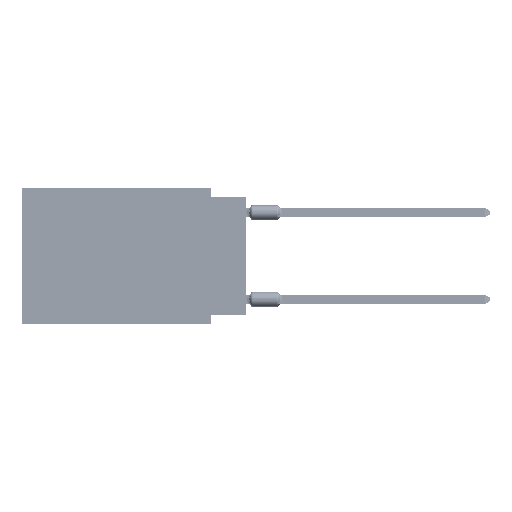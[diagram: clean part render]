
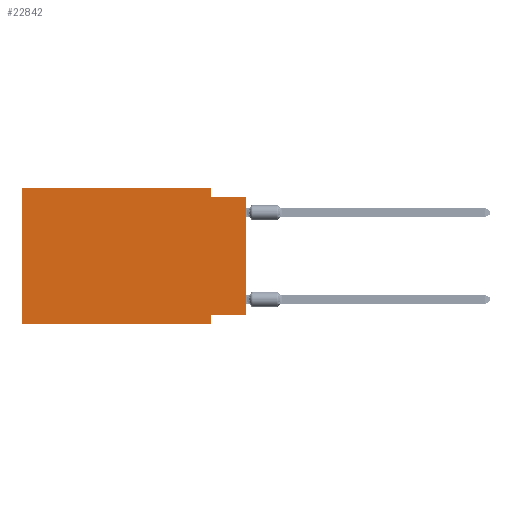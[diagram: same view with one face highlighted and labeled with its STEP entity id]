
A CAD part, left-side view. The second image highlights one B-rep face of the part: STEP entity #22842.
In plain terms, the highlighted planar face has unit normal (-1, 0, 0).
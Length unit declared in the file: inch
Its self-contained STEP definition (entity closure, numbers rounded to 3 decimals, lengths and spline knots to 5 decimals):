
#12 = VERTEX_POINT ( 'NONE', #15756 ) ;
#112 = FACE_OUTER_BOUND ( 'NONE', #55734, .T. ) ;
#327 = EDGE_CURVE ( 'NONE', #12, #71930, #74552, .T. ) ;
#1677 = DIRECTION ( 'NONE',  ( 0., 0., -1. ) ) ;
#2386 = ORIENTED_EDGE ( 'NONE', *, *, #60859, .T. ) ;
#9973 = CARTESIAN_POINT ( 'NONE',  ( 0., 0.645, -0.39 ) ) ;
#10637 = CARTESIAN_POINT ( 'NONE',  ( 0., 0.1, 0. ) ) ;
#10812 = VECTOR ( 'NONE', #62436, 39.37008 ) ;
#10823 = EDGE_CURVE ( 'NONE', #30338, #66851, #62764, .T. ) ;
#11741 = LINE ( 'NONE', #49872, #10812 ) ;
#14947 = CARTESIAN_POINT ( 'NONE',  ( 0., 0.645, 0. ) ) ;
#15350 = LINE ( 'NONE', #14947, #48545 ) ;
#15441 = VECTOR ( 'NONE', #75757, 39.37008 ) ;
#15746 = ORIENTED_EDGE ( 'NONE', *, *, #327, .F. ) ;
#15756 = CARTESIAN_POINT ( 'NONE',  ( 0., 0.1, -0.025 ) ) ;
#17090 = EDGE_CURVE ( 'NONE', #29389, #30338, #11741, .T. ) ;
#18115 = LINE ( 'NONE', #48184, #34648 ) ;
#18523 = EDGE_CURVE ( 'NONE', #76039, #56901, #15350, .T. ) ;
#19730 = CARTESIAN_POINT ( 'NONE',  ( 0., 0.1, -0.365 ) ) ;
#22842 = ADVANCED_FACE ( 'NONE', ( #112 ), #74008, .F. ) ;
#25514 = CARTESIAN_POINT ( 'NONE',  ( 0., 0.645, 0. ) ) ;
#29389 = VERTEX_POINT ( 'NONE', #50410 ) ;
#30338 = VERTEX_POINT ( 'NONE', #19730 ) ;
#30595 = CARTESIAN_POINT ( 'NONE',  ( 0., 0.645, -0.39 ) ) ;
#31672 = CARTESIAN_POINT ( 'NONE',  ( 0., 0.645, 0. ) ) ;
#32279 = EDGE_CURVE ( 'NONE', #56901, #12, #40653, .T. ) ;
#32532 = CARTESIAN_POINT ( 'NONE',  ( 0., 0.1, 0. ) ) ;
#33145 = VECTOR ( 'NONE', #62234, 39.37008 ) ;
#34553 = AXIS2_PLACEMENT_3D ( 'NONE', #41994, #73611, #61027 ) ;
#34648 = VECTOR ( 'NONE', #55455, 39.37008 ) ;
#34811 = CARTESIAN_POINT ( 'NONE',  ( 0., 0.1, -0.39 ) ) ;
#35458 = VECTOR ( 'NONE', #62369, 39.37008 ) ;
#40653 = LINE ( 'NONE', #32532, #79321 ) ;
#41693 = VERTEX_POINT ( 'NONE', #9973 ) ;
#41994 = CARTESIAN_POINT ( 'NONE',  ( 0., 0.645, 0. ) ) ;
#43728 = CARTESIAN_POINT ( 'NONE',  ( 0., 0., -0.025 ) ) ;
#48184 = CARTESIAN_POINT ( 'NONE',  ( 0., 0., 0. ) ) ;
#48318 = ORIENTED_EDGE ( 'NONE', *, *, #32279, .F. ) ;
#48476 = LINE ( 'NONE', #30595, #33145 ) ;
#48545 = VECTOR ( 'NONE', #64445, 39.37008 ) ;
#49872 = CARTESIAN_POINT ( 'NONE',  ( 0., 0., -0.365 ) ) ;
#50410 = CARTESIAN_POINT ( 'NONE',  ( 0., 0., -0.365 ) ) ;
#50679 = DIRECTION ( 'NONE',  ( 0., 0., 1. ) ) ;
#51680 = ORIENTED_EDGE ( 'NONE', *, *, #62067, .T. ) ;
#55455 = DIRECTION ( 'NONE',  ( 0., 0., 1. ) ) ;
#55734 = EDGE_LOOP ( 'NONE', ( #51680, #15746, #48318, #72112, #73805, #2386, #66649, #71042 ) ) ;
#56901 = VERTEX_POINT ( 'NONE', #10637 ) ;
#60859 = EDGE_CURVE ( 'NONE', #41693, #66851, #48476, .T. ) ;
#61027 = DIRECTION ( 'NONE',  ( 0., 0., -1. ) ) ;
#62067 = EDGE_CURVE ( 'NONE', #29389, #71930, #18115, .T. ) ;
#62234 = DIRECTION ( 'NONE',  ( 0., -1., 0. ) ) ;
#62369 = DIRECTION ( 'NONE',  ( 0., -1., 0. ) ) ;
#62436 = DIRECTION ( 'NONE',  ( 0., 1., 0. ) ) ;
#62525 = VECTOR ( 'NONE', #50679, 39.37008 ) ;
#62764 = LINE ( 'NONE', #76159, #15441 ) ;
#64201 = CARTESIAN_POINT ( 'NONE',  ( 0., 0., -0.025 ) ) ;
#64445 = DIRECTION ( 'NONE',  ( 0., -1., 0. ) ) ;
#66649 = ORIENTED_EDGE ( 'NONE', *, *, #10823, .F. ) ;
#66851 = VERTEX_POINT ( 'NONE', #34811 ) ;
#70776 = EDGE_CURVE ( 'NONE', #41693, #76039, #75429, .T. ) ;
#71042 = ORIENTED_EDGE ( 'NONE', *, *, #17090, .F. ) ;
#71930 = VERTEX_POINT ( 'NONE', #64201 ) ;
#72112 = ORIENTED_EDGE ( 'NONE', *, *, #18523, .F. ) ;
#73611 = DIRECTION ( 'NONE',  ( 1., 0., 0. ) ) ;
#73805 = ORIENTED_EDGE ( 'NONE', *, *, #70776, .F. ) ;
#74008 = PLANE ( 'NONE',  #34553 ) ;
#74552 = LINE ( 'NONE', #43728, #35458 ) ;
#75429 = LINE ( 'NONE', #25514, #62525 ) ;
#75757 = DIRECTION ( 'NONE',  ( 0., 0., -1. ) ) ;
#76039 = VERTEX_POINT ( 'NONE', #31672 ) ;
#76159 = CARTESIAN_POINT ( 'NONE',  ( 0., 0.1, -0.39 ) ) ;
#79321 = VECTOR ( 'NONE', #1677, 39.37008 ) ;
